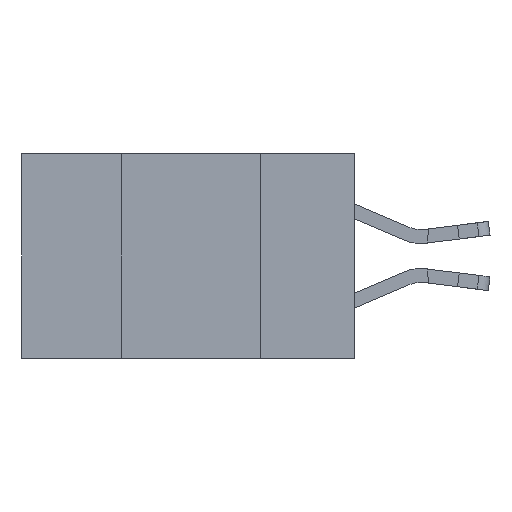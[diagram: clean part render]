
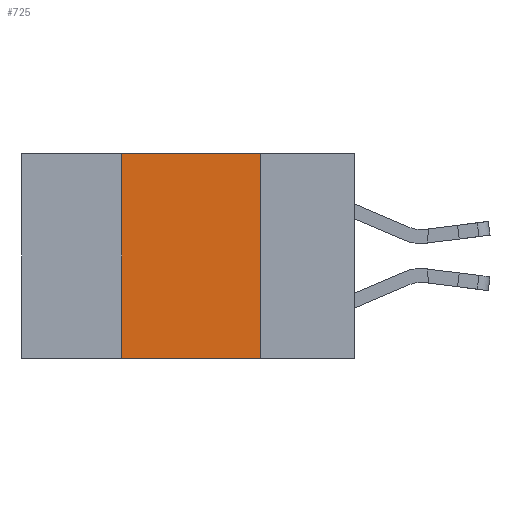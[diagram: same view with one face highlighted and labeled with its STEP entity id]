
A CAD part, left-side view. The second image highlights one B-rep face of the part: STEP entity #725.
In plain terms, the highlighted planar face has unit normal (-1, 0, 0).
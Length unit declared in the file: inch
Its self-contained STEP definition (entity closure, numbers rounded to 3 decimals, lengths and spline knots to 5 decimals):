
#570 = VECTOR ( 'NONE', #3988, 39.37008 ) ;
#725 = ADVANCED_FACE ( 'NONE', ( #11483 ), #10591, .F. ) ;
#874 = VERTEX_POINT ( 'NONE', #1710 ) ;
#1415 = LINE ( 'NONE', #10637, #3824 ) ;
#1580 = ORIENTED_EDGE ( 'NONE', *, *, #7792, .F. ) ;
#1710 = CARTESIAN_POINT ( 'NONE',  ( 0., 0.17, 0. ) ) ;
#2705 = VERTEX_POINT ( 'NONE', #5393 ) ;
#3223 = DIRECTION ( 'NONE',  ( 0., 0., -1. ) ) ;
#3320 = CARTESIAN_POINT ( 'NONE',  ( 0., 0.42, -0.37 ) ) ;
#3352 = EDGE_CURVE ( 'NONE', #7262, #2705, #8307, .T. ) ;
#3450 = VECTOR ( 'NONE', #3223, 39.37008 ) ;
#3690 = AXIS2_PLACEMENT_3D ( 'NONE', #11204, #7435, #7341 ) ;
#3824 = VECTOR ( 'NONE', #10676, 39.37008 ) ;
#3941 = CARTESIAN_POINT ( 'NONE',  ( 0., 0.17, 0. ) ) ;
#3988 = DIRECTION ( 'NONE',  ( 0., 0., 1. ) ) ;
#4031 = VECTOR ( 'NONE', #6714, 39.37008 ) ;
#4056 = EDGE_CURVE ( 'NONE', #7262, #8878, #1415, .T. ) ;
#4096 = EDGE_LOOP ( 'NONE', ( #9707, #1580, #5859, #8940 ) ) ;
#5393 = CARTESIAN_POINT ( 'NONE',  ( 0., 0.42, 0. ) ) ;
#5557 = CARTESIAN_POINT ( 'NONE',  ( 0., 0.42, 0. ) ) ;
#5700 = EDGE_CURVE ( 'NONE', #874, #8878, #10769, .T. ) ;
#5859 = ORIENTED_EDGE ( 'NONE', *, *, #3352, .F. ) ;
#6214 = LINE ( 'NONE', #12183, #4031 ) ;
#6714 = DIRECTION ( 'NONE',  ( 0., -1., 0. ) ) ;
#7262 = VERTEX_POINT ( 'NONE', #3320 ) ;
#7341 = DIRECTION ( 'NONE',  ( 0., 0., -1. ) ) ;
#7435 = DIRECTION ( 'NONE',  ( 1., 0., 0. ) ) ;
#7792 = EDGE_CURVE ( 'NONE', #2705, #874, #6214, .T. ) ;
#8307 = LINE ( 'NONE', #5557, #570 ) ;
#8878 = VERTEX_POINT ( 'NONE', #11546 ) ;
#8940 = ORIENTED_EDGE ( 'NONE', *, *, #4056, .T. ) ;
#9707 = ORIENTED_EDGE ( 'NONE', *, *, #5700, .F. ) ;
#10591 = PLANE ( 'NONE',  #3690 ) ;
#10637 = CARTESIAN_POINT ( 'NONE',  ( 0., 0.6, -0.37 ) ) ;
#10676 = DIRECTION ( 'NONE',  ( 0., -1., 0. ) ) ;
#10769 = LINE ( 'NONE', #3941, #3450 ) ;
#11204 = CARTESIAN_POINT ( 'NONE',  ( 0., 0.6, 0. ) ) ;
#11483 = FACE_OUTER_BOUND ( 'NONE', #4096, .T. ) ;
#11546 = CARTESIAN_POINT ( 'NONE',  ( 0., 0.17, -0.37 ) ) ;
#12183 = CARTESIAN_POINT ( 'NONE',  ( 0., 0.6, 0. ) ) ;
